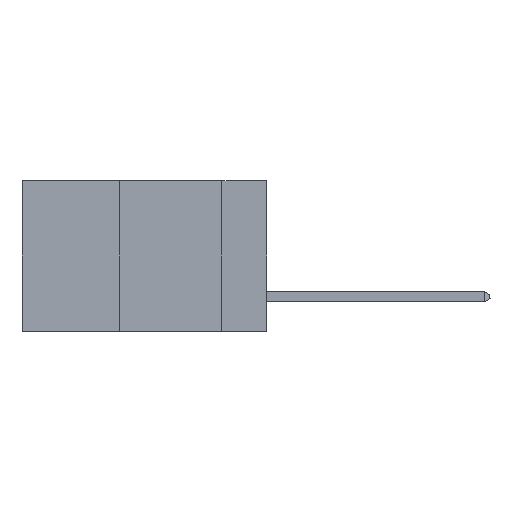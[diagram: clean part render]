
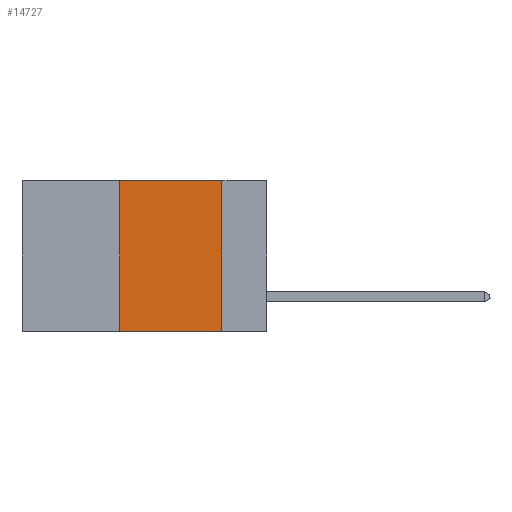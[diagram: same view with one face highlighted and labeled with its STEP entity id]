
A CAD part, left-side view. The second image highlights one B-rep face of the part: STEP entity #14727.
In plain terms, the highlighted planar face has unit normal (-1, 0, 0).
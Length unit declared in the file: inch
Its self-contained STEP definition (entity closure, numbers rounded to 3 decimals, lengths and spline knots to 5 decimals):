
#246 = CARTESIAN_POINT ( 'NONE',  ( 0., 0.6, 0. ) ) ;
#385 = CARTESIAN_POINT ( 'NONE',  ( 0., 0.11, -0.37 ) ) ;
#399 = CARTESIAN_POINT ( 'NONE',  ( 0., 0.6, 0. ) ) ;
#761 = DIRECTION ( 'NONE',  ( 0., 0., -1. ) ) ;
#1448 = EDGE_CURVE ( 'NONE', #8638, #21232, #19613, .T. ) ;
#2092 = EDGE_LOOP ( 'NONE', ( #16519, #4846, #9490, #12508 ) ) ;
#2335 = LINE ( 'NONE', #12794, #19056 ) ;
#2505 = CARTESIAN_POINT ( 'NONE',  ( 0., 0.11, 0. ) ) ;
#4650 = VECTOR ( 'NONE', #20731, 39.37008 ) ;
#4712 = CARTESIAN_POINT ( 'NONE',  ( 0., 0.11, 0. ) ) ;
#4846 = ORIENTED_EDGE ( 'NONE', *, *, #14759, .F. ) ;
#5105 = VECTOR ( 'NONE', #18731, 39.37008 ) ;
#5149 = CARTESIAN_POINT ( 'NONE',  ( 0., 0.36, 0. ) ) ;
#5531 = DIRECTION ( 'NONE',  ( 1., 0., 0. ) ) ;
#5554 = AXIS2_PLACEMENT_3D ( 'NONE', #399, #5531, #761 ) ;
#8363 = PLANE ( 'NONE',  #5554 ) ;
#8638 = VERTEX_POINT ( 'NONE', #2505 ) ;
#9490 = ORIENTED_EDGE ( 'NONE', *, *, #19353, .F. ) ;
#10415 = VECTOR ( 'NONE', #13325, 39.37008 ) ;
#12271 = EDGE_CURVE ( 'NONE', #20367, #21232, #13389, .T. ) ;
#12508 = ORIENTED_EDGE ( 'NONE', *, *, #12271, .T. ) ;
#12726 = DIRECTION ( 'NONE',  ( 0., 0., 1. ) ) ;
#12794 = CARTESIAN_POINT ( 'NONE',  ( 0., 0.36, 0. ) ) ;
#13325 = DIRECTION ( 'NONE',  ( 0., 0., -1. ) ) ;
#13389 = LINE ( 'NONE', #15189, #4650 ) ;
#14727 = ADVANCED_FACE ( 'NONE', ( #15913 ), #8363, .F. ) ;
#14759 = EDGE_CURVE ( 'NONE', #20403, #8638, #20724, .T. ) ;
#15189 = CARTESIAN_POINT ( 'NONE',  ( 0., 0.6, -0.37 ) ) ;
#15651 = CARTESIAN_POINT ( 'NONE',  ( 0., 0.36, -0.37 ) ) ;
#15913 = FACE_OUTER_BOUND ( 'NONE', #2092, .T. ) ;
#16519 = ORIENTED_EDGE ( 'NONE', *, *, #1448, .F. ) ;
#18731 = DIRECTION ( 'NONE',  ( 0., -1., 0. ) ) ;
#19056 = VECTOR ( 'NONE', #12726, 39.37008 ) ;
#19353 = EDGE_CURVE ( 'NONE', #20367, #20403, #2335, .T. ) ;
#19613 = LINE ( 'NONE', #4712, #10415 ) ;
#20367 = VERTEX_POINT ( 'NONE', #15651 ) ;
#20403 = VERTEX_POINT ( 'NONE', #5149 ) ;
#20724 = LINE ( 'NONE', #246, #5105 ) ;
#20731 = DIRECTION ( 'NONE',  ( 0., -1., 0. ) ) ;
#21232 = VERTEX_POINT ( 'NONE', #385 ) ;
